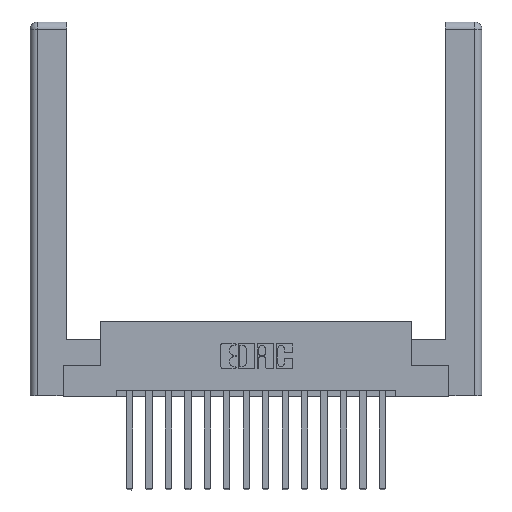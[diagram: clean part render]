
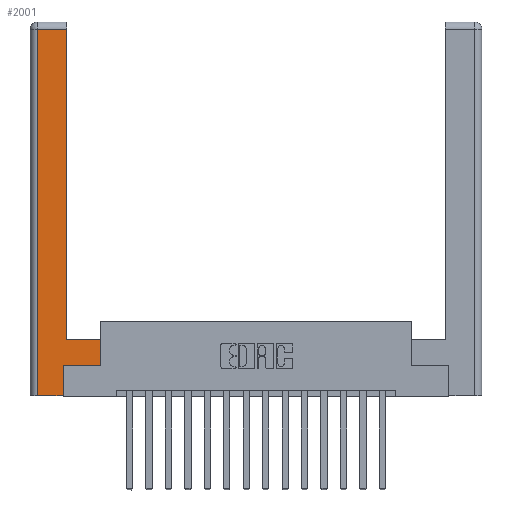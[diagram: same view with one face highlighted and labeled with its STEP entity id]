
A CAD part, top view. The second image highlights one B-rep face of the part: STEP entity #2001.
In plain terms, the highlighted planar face has unit normal (0, 0, 1).
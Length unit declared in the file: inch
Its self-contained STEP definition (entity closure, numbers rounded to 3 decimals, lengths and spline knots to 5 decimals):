
#98 = VECTOR ( 'NONE', #9967, 39.37008 ) ;
#354 = EDGE_CURVE ( 'NONE', #13714, #12105, #6981, .T. ) ;
#444 = LINE ( 'NONE', #7838, #11470 ) ;
#466 = DIRECTION ( 'NONE',  ( -1., 0., 0. ) ) ;
#540 = CARTESIAN_POINT ( 'NONE',  ( 0.565, 0.45, 0. ) ) ;
#1381 = EDGE_CURVE ( 'NONE', #15861, #11311, #6539, .T. ) ;
#1577 = DIRECTION ( 'NONE',  ( 1., 0., 0. ) ) ;
#2001 = ADVANCED_FACE ( 'NONE', ( #13885 ), #6970, .F. ) ;
#2173 = LINE ( 'NONE', #11445, #98 ) ;
#2534 = CARTESIAN_POINT ( 'NONE',  ( 0.265, 0., 0. ) ) ;
#2754 = CARTESIAN_POINT ( 'NONE',  ( 0.295, 0.45, 0. ) ) ;
#2920 = LINE ( 'NONE', #14851, #4158 ) ;
#3041 = CARTESIAN_POINT ( 'NONE',  ( 0., 0., 0. ) ) ;
#3945 = CARTESIAN_POINT ( 'NONE',  ( 0.0615, 2.94, 0. ) ) ;
#4122 = EDGE_LOOP ( 'NONE', ( #8308, #16703, #4165, #5388, #8733, #5663, #5390, #12646 ) ) ;
#4158 = VECTOR ( 'NONE', #1577, 39.37008 ) ;
#4165 = ORIENTED_EDGE ( 'NONE', *, *, #13198, .T. ) ;
#4351 = VECTOR ( 'NONE', #11556, 39.37008 ) ;
#4371 = DIRECTION ( 'NONE',  ( 0., 0., -1. ) ) ;
#4577 = AXIS2_PLACEMENT_3D ( 'NONE', #3041, #4371, #466 ) ;
#4764 = VECTOR ( 'NONE', #8243, 39.37008 ) ;
#5388 = ORIENTED_EDGE ( 'NONE', *, *, #354, .T. ) ;
#5390 = ORIENTED_EDGE ( 'NONE', *, *, #16475, .T. ) ;
#5663 = ORIENTED_EDGE ( 'NONE', *, *, #7118, .T. ) ;
#5695 = CARTESIAN_POINT ( 'NONE',  ( 0.265, 0.245, 0. ) ) ;
#5957 = VERTEX_POINT ( 'NONE', #3945 ) ;
#6539 = LINE ( 'NONE', #2754, #13906 ) ;
#6741 = DIRECTION ( 'NONE',  ( -1., 0., 0. ) ) ;
#6970 = PLANE ( 'NONE',  #4577 ) ;
#6981 = LINE ( 'NONE', #2534, #4351 ) ;
#7118 = EDGE_CURVE ( 'NONE', #12393, #10558, #2920, .T. ) ;
#7198 = DIRECTION ( 'NONE',  ( 0., -1., 0. ) ) ;
#7231 = EDGE_CURVE ( 'NONE', #11311, #13520, #11714, .T. ) ;
#7323 = CARTESIAN_POINT ( 'NONE',  ( 0.265, 0.245, 0. ) ) ;
#7698 = EDGE_CURVE ( 'NONE', #13520, #5957, #444, .T. ) ;
#7838 = CARTESIAN_POINT ( 'NONE',  ( 0.0615, 2.94, 0. ) ) ;
#8243 = DIRECTION ( 'NONE',  ( 0., 1., 0. ) ) ;
#8308 = ORIENTED_EDGE ( 'NONE', *, *, #7231, .T. ) ;
#8733 = ORIENTED_EDGE ( 'NONE', *, *, #11750, .T. ) ;
#8776 = CARTESIAN_POINT ( 'NONE',  ( 0.295, 0.45, 0. ) ) ;
#9967 = DIRECTION ( 'NONE',  ( 0., 1., 0. ) ) ;
#10558 = VERTEX_POINT ( 'NONE', #14062 ) ;
#11311 = VERTEX_POINT ( 'NONE', #8776 ) ;
#11445 = CARTESIAN_POINT ( 'NONE',  ( 0.565, 0.45, 0. ) ) ;
#11470 = VECTOR ( 'NONE', #6741, 39.37008 ) ;
#11556 = DIRECTION ( 'NONE',  ( 1., 0., 0. ) ) ;
#11714 = LINE ( 'NONE', #13288, #4764 ) ;
#11750 = EDGE_CURVE ( 'NONE', #12105, #12393, #12969, .T. ) ;
#11936 = VECTOR ( 'NONE', #15123, 39.37008 ) ;
#12105 = VERTEX_POINT ( 'NONE', #14154 ) ;
#12393 = VERTEX_POINT ( 'NONE', #5695 ) ;
#12423 = CARTESIAN_POINT ( 'NONE',  ( 0.0615, 0., 0. ) ) ;
#12646 = ORIENTED_EDGE ( 'NONE', *, *, #1381, .T. ) ;
#12969 = LINE ( 'NONE', #7323, #11936 ) ;
#13197 = DIRECTION ( 'NONE',  ( -1., 0., 0. ) ) ;
#13198 = EDGE_CURVE ( 'NONE', #5957, #13714, #14346, .T. ) ;
#13288 = CARTESIAN_POINT ( 'NONE',  ( 0.295, 3., 0. ) ) ;
#13304 = CARTESIAN_POINT ( 'NONE',  ( 0.295, 2.94, 0. ) ) ;
#13520 = VERTEX_POINT ( 'NONE', #13304 ) ;
#13594 = CARTESIAN_POINT ( 'NONE',  ( 0.0615, 0., 0. ) ) ;
#13714 = VERTEX_POINT ( 'NONE', #13594 ) ;
#13885 = FACE_OUTER_BOUND ( 'NONE', #4122, .T. ) ;
#13906 = VECTOR ( 'NONE', #13197, 39.37008 ) ;
#14062 = CARTESIAN_POINT ( 'NONE',  ( 0.565, 0.245, 0. ) ) ;
#14154 = CARTESIAN_POINT ( 'NONE',  ( 0.265, 0., 0. ) ) ;
#14346 = LINE ( 'NONE', #12423, #15182 ) ;
#14851 = CARTESIAN_POINT ( 'NONE',  ( 0.565, 0.245, 0. ) ) ;
#15123 = DIRECTION ( 'NONE',  ( 0., 1., 0. ) ) ;
#15182 = VECTOR ( 'NONE', #7198, 39.37008 ) ;
#15861 = VERTEX_POINT ( 'NONE', #540 ) ;
#16475 = EDGE_CURVE ( 'NONE', #10558, #15861, #2173, .T. ) ;
#16703 = ORIENTED_EDGE ( 'NONE', *, *, #7698, .T. ) ;
